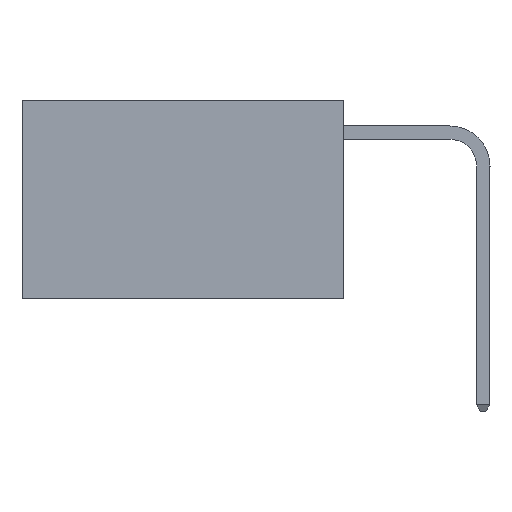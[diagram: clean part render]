
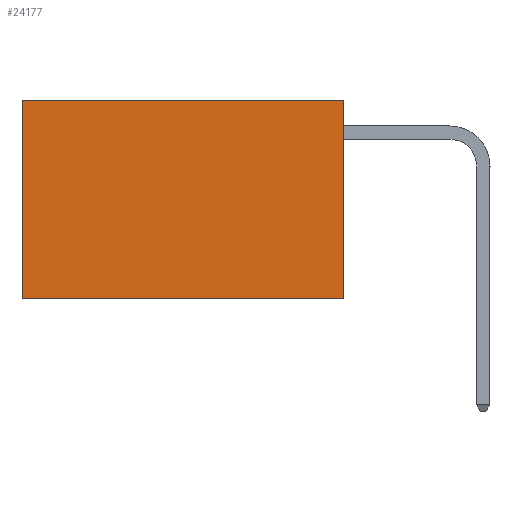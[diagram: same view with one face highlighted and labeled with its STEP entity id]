
A CAD part, left-side view. The second image highlights one B-rep face of the part: STEP entity #24177.
In plain terms, the highlighted planar face has unit normal (-1, 0, 0).
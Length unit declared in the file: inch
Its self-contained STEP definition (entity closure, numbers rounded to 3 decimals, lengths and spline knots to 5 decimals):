
#109 = DIRECTION ( 'NONE',  ( 0., 0., -1. ) ) ;
#527 = CARTESIAN_POINT ( 'NONE',  ( 0.2625, 0., 0. ) ) ;
#1195 = CARTESIAN_POINT ( 'NONE',  ( 0.2625, 0., 0. ) ) ;
#2180 = VECTOR ( 'NONE', #10840, 39.37008 ) ;
#2822 = LINE ( 'NONE', #8783, #2180 ) ;
#3144 = EDGE_LOOP ( 'NONE', ( #8041, #5416, #22617, #11391 ) ) ;
#3428 = CARTESIAN_POINT ( 'NONE',  ( 0.2625, 0.6, 0. ) ) ;
#4194 = CARTESIAN_POINT ( 'NONE',  ( 0.2625, 0.6, 0. ) ) ;
#4372 = CARTESIAN_POINT ( 'NONE',  ( 0.2625, 0., 0. ) ) ;
#5315 = EDGE_CURVE ( 'NONE', #26058, #12828, #6519, .T. ) ;
#5320 = PLANE ( 'NONE',  #16625 ) ;
#5416 = ORIENTED_EDGE ( 'NONE', *, *, #22275, .F. ) ;
#6519 = LINE ( 'NONE', #12691, #22031 ) ;
#7368 = DIRECTION ( 'NONE',  ( 0., 0., -1. ) ) ;
#8041 = ORIENTED_EDGE ( 'NONE', *, *, #25162, .T. ) ;
#8503 = LINE ( 'NONE', #527, #24020 ) ;
#8580 = CARTESIAN_POINT ( 'NONE',  ( 0.2625, 0., -0.37 ) ) ;
#8783 = CARTESIAN_POINT ( 'NONE',  ( 0.2625, 0., -0.37 ) ) ;
#9113 = FACE_OUTER_BOUND ( 'NONE', #3144, .T. ) ;
#10749 = VERTEX_POINT ( 'NONE', #19073 ) ;
#10840 = DIRECTION ( 'NONE',  ( 0., 1., 0. ) ) ;
#10945 = VECTOR ( 'NONE', #109, 39.37008 ) ;
#11391 = ORIENTED_EDGE ( 'NONE', *, *, #19159, .T. ) ;
#12691 = CARTESIAN_POINT ( 'NONE',  ( 0.2625, 0., 0. ) ) ;
#12828 = VERTEX_POINT ( 'NONE', #8580 ) ;
#14744 = DIRECTION ( 'NONE',  ( 0., 0., -1. ) ) ;
#16625 = AXIS2_PLACEMENT_3D ( 'NONE', #1195, #19472, #7368 ) ;
#18679 = DIRECTION ( 'NONE',  ( 0., 1., 0. ) ) ;
#19073 = CARTESIAN_POINT ( 'NONE',  ( 0.2625, 0.6, -0.37 ) ) ;
#19159 = EDGE_CURVE ( 'NONE', #26058, #22569, #8503, .T. ) ;
#19472 = DIRECTION ( 'NONE',  ( 1., 0., 0. ) ) ;
#21679 = LINE ( 'NONE', #4194, #10945 ) ;
#22031 = VECTOR ( 'NONE', #14744, 39.37008 ) ;
#22275 = EDGE_CURVE ( 'NONE', #12828, #10749, #2822, .T. ) ;
#22569 = VERTEX_POINT ( 'NONE', #3428 ) ;
#22617 = ORIENTED_EDGE ( 'NONE', *, *, #5315, .F. ) ;
#24020 = VECTOR ( 'NONE', #18679, 39.37008 ) ;
#24177 = ADVANCED_FACE ( 'NONE', ( #9113 ), #5320, .F. ) ;
#25162 = EDGE_CURVE ( 'NONE', #22569, #10749, #21679, .T. ) ;
#26058 = VERTEX_POINT ( 'NONE', #4372 ) ;
